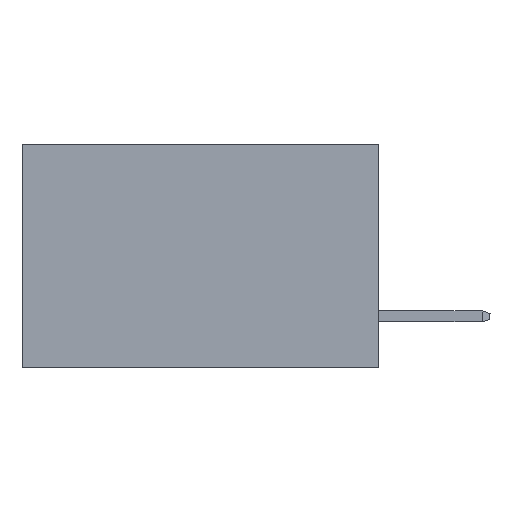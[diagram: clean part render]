
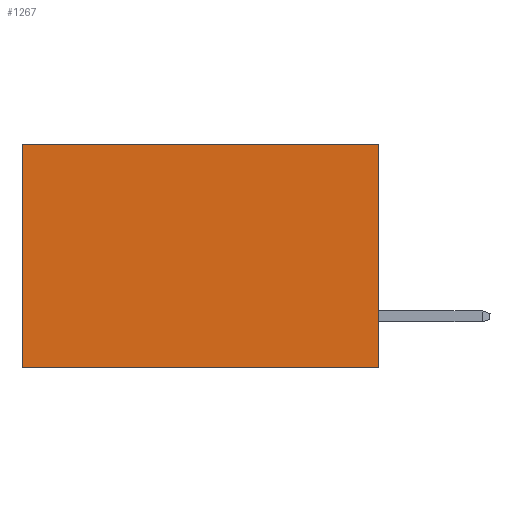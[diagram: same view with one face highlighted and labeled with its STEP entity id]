
A CAD part, left-side view. The second image highlights one B-rep face of the part: STEP entity #1267.
In plain terms, the highlighted planar face has unit normal (-1, 0, 0).
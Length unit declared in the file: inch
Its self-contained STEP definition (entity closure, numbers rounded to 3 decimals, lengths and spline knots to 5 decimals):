
#335 = VECTOR ( 'NONE', #10292, 39.37008 ) ;
#472 = VERTEX_POINT ( 'NONE', #12643 ) ;
#615 = DIRECTION ( 'NONE',  ( 0., 0., -1. ) ) ;
#1267 = ADVANCED_FACE ( 'NONE', ( #11944 ), #2802, .F. ) ;
#1500 = ORIENTED_EDGE ( 'NONE', *, *, #6903, .T. ) ;
#1614 = DIRECTION ( 'NONE',  ( 0., 1., 0. ) ) ;
#1714 = EDGE_CURVE ( 'NONE', #12370, #11017, #4502, .T. ) ;
#2308 = LINE ( 'NONE', #8039, #7260 ) ;
#2802 = PLANE ( 'NONE',  #3034 ) ;
#3023 = CARTESIAN_POINT ( 'NONE',  ( 0.277, 0., -0.37 ) ) ;
#3034 = AXIS2_PLACEMENT_3D ( 'NONE', #8493, #5354, #615 ) ;
#4086 = VERTEX_POINT ( 'NONE', #8662 ) ;
#4455 = LINE ( 'NONE', #8497, #9638 ) ;
#4502 = LINE ( 'NONE', #3023, #9389 ) ;
#4746 = LINE ( 'NONE', #10544, #335 ) ;
#5185 = DIRECTION ( 'NONE',  ( 0., 0., -1. ) ) ;
#5354 = DIRECTION ( 'NONE',  ( 1., 0., 0. ) ) ;
#5826 = EDGE_LOOP ( 'NONE', ( #1500, #9337, #7068, #9625 ) ) ;
#6903 = EDGE_CURVE ( 'NONE', #4086, #472, #4746, .T. ) ;
#7068 = ORIENTED_EDGE ( 'NONE', *, *, #1714, .F. ) ;
#7260 = VECTOR ( 'NONE', #7991, 39.37008 ) ;
#7740 = CARTESIAN_POINT ( 'NONE',  ( 0.277, 0., -0.37 ) ) ;
#7991 = DIRECTION ( 'NONE',  ( 0., 1., 0. ) ) ;
#8039 = CARTESIAN_POINT ( 'NONE',  ( 0.277, 0., -0.37 ) ) ;
#8493 = CARTESIAN_POINT ( 'NONE',  ( 0.277, 0., -0.37 ) ) ;
#8497 = CARTESIAN_POINT ( 'NONE',  ( 0.277, 0., 0. ) ) ;
#8662 = CARTESIAN_POINT ( 'NONE',  ( 0.277, 0.59, 0. ) ) ;
#9337 = ORIENTED_EDGE ( 'NONE', *, *, #9399, .F. ) ;
#9389 = VECTOR ( 'NONE', #5185, 39.37008 ) ;
#9399 = EDGE_CURVE ( 'NONE', #11017, #472, #2308, .T. ) ;
#9625 = ORIENTED_EDGE ( 'NONE', *, *, #12310, .T. ) ;
#9638 = VECTOR ( 'NONE', #1614, 39.37008 ) ;
#10292 = DIRECTION ( 'NONE',  ( 0., 0., -1. ) ) ;
#10544 = CARTESIAN_POINT ( 'NONE',  ( 0.277, 0.59, -0.37 ) ) ;
#11017 = VERTEX_POINT ( 'NONE', #7740 ) ;
#11450 = CARTESIAN_POINT ( 'NONE',  ( 0.277, 0., 0. ) ) ;
#11944 = FACE_OUTER_BOUND ( 'NONE', #5826, .T. ) ;
#12310 = EDGE_CURVE ( 'NONE', #12370, #4086, #4455, .T. ) ;
#12370 = VERTEX_POINT ( 'NONE', #11450 ) ;
#12643 = CARTESIAN_POINT ( 'NONE',  ( 0.277, 0.59, -0.37 ) ) ;
